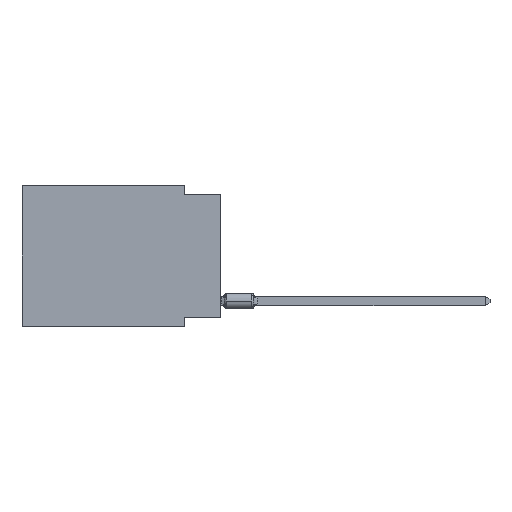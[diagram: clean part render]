
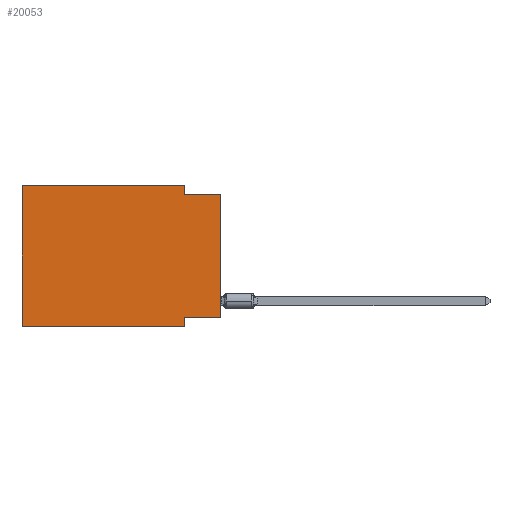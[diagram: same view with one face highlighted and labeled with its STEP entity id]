
A CAD part, left-side view. The second image highlights one B-rep face of the part: STEP entity #20053.
In plain terms, the highlighted planar face has unit normal (-1, 0, 0).
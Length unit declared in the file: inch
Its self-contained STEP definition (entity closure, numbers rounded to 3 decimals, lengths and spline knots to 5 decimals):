
#41 = EDGE_CURVE ( 'NONE', #33202, #29079, #17426, .T. ) ;
#265 = LINE ( 'NONE', #12727, #940 ) ;
#940 = VECTOR ( 'NONE', #28941, 39.37008 ) ;
#988 = CARTESIAN_POINT ( 'NONE',  ( 0., 0., -0.025 ) ) ;
#1193 = VECTOR ( 'NONE', #3491, 39.37008 ) ;
#2106 = AXIS2_PLACEMENT_3D ( 'NONE', #7071, #19017, #40010 ) ;
#3491 = DIRECTION ( 'NONE',  ( 0., 1., 0. ) ) ;
#4586 = VERTEX_POINT ( 'NONE', #39577 ) ;
#5908 = CARTESIAN_POINT ( 'NONE',  ( 0., 0., 0. ) ) ;
#7071 = CARTESIAN_POINT ( 'NONE',  ( 0., 0.55, 0. ) ) ;
#7838 = ORIENTED_EDGE ( 'NONE', *, *, #26029, .F. ) ;
#7906 = ORIENTED_EDGE ( 'NONE', *, *, #47358, .T. ) ;
#8209 = VERTEX_POINT ( 'NONE', #19901 ) ;
#10557 = DIRECTION ( 'NONE',  ( 0., -1., 0. ) ) ;
#10739 = CARTESIAN_POINT ( 'NONE',  ( 0., 0.1, -0.025 ) ) ;
#11230 = EDGE_CURVE ( 'NONE', #8209, #22387, #38913, .T. ) ;
#11458 = VECTOR ( 'NONE', #20767, 39.37008 ) ;
#12727 = CARTESIAN_POINT ( 'NONE',  ( 0., 0.1, 0. ) ) ;
#13503 = VECTOR ( 'NONE', #10557, 39.37008 ) ;
#15391 = EDGE_CURVE ( 'NONE', #31504, #23807, #30764, .T. ) ;
#16105 = VECTOR ( 'NONE', #34143, 39.37008 ) ;
#16266 = CARTESIAN_POINT ( 'NONE',  ( 0., 0.55, -0.39 ) ) ;
#17426 = LINE ( 'NONE', #988, #40096 ) ;
#17578 = DIRECTION ( 'NONE',  ( 0., 0., 1. ) ) ;
#19017 = DIRECTION ( 'NONE',  ( 1., 0., 0. ) ) ;
#19901 = CARTESIAN_POINT ( 'NONE',  ( 0., 0.55, 0. ) ) ;
#19942 = LINE ( 'NONE', #40395, #1193 ) ;
#20053 = ADVANCED_FACE ( 'NONE', ( #27281 ), #23029, .F. ) ;
#20767 = DIRECTION ( 'NONE',  ( 0., 0., 1. ) ) ;
#22218 = CARTESIAN_POINT ( 'NONE',  ( 0., 0.1, -0.39 ) ) ;
#22387 = VERTEX_POINT ( 'NONE', #44448 ) ;
#23029 = PLANE ( 'NONE',  #2106 ) ;
#23807 = VERTEX_POINT ( 'NONE', #52508 ) ;
#24444 = ORIENTED_EDGE ( 'NONE', *, *, #41, .F. ) ;
#25824 = LINE ( 'NONE', #5908, #42724 ) ;
#26029 = EDGE_CURVE ( 'NONE', #4586, #26253, #19942, .T. ) ;
#26253 = VERTEX_POINT ( 'NONE', #43676 ) ;
#27281 = FACE_OUTER_BOUND ( 'NONE', #33804, .T. ) ;
#28511 = CARTESIAN_POINT ( 'NONE',  ( 0., 0., -0.025 ) ) ;
#28941 = DIRECTION ( 'NONE',  ( 0., 0., -1. ) ) ;
#29079 = VERTEX_POINT ( 'NONE', #28511 ) ;
#30367 = EDGE_CURVE ( 'NONE', #31504, #8209, #37250, .T. ) ;
#30508 = CARTESIAN_POINT ( 'NONE',  ( 0., 0.55, -0.39 ) ) ;
#30764 = LINE ( 'NONE', #30508, #13503 ) ;
#31504 = VERTEX_POINT ( 'NONE', #16266 ) ;
#33202 = VERTEX_POINT ( 'NONE', #10739 ) ;
#33263 = ORIENTED_EDGE ( 'NONE', *, *, #15391, .T. ) ;
#33804 = EDGE_LOOP ( 'NONE', ( #7906, #24444, #36402, #45038, #39107, #33263, #42255, #7838 ) ) ;
#34143 = DIRECTION ( 'NONE',  ( 0., -1., 0. ) ) ;
#35199 = VECTOR ( 'NONE', #38928, 39.37008 ) ;
#36402 = ORIENTED_EDGE ( 'NONE', *, *, #41595, .F. ) ;
#37113 = DIRECTION ( 'NONE',  ( 0., -1., 0. ) ) ;
#37250 = LINE ( 'NONE', #44949, #11458 ) ;
#38647 = CARTESIAN_POINT ( 'NONE',  ( 0., 0.55, 0. ) ) ;
#38913 = LINE ( 'NONE', #38647, #16105 ) ;
#38928 = DIRECTION ( 'NONE',  ( 0., 0., -1. ) ) ;
#39107 = ORIENTED_EDGE ( 'NONE', *, *, #30367, .F. ) ;
#39190 = LINE ( 'NONE', #22218, #35199 ) ;
#39577 = CARTESIAN_POINT ( 'NONE',  ( 0., 0., -0.365 ) ) ;
#40010 = DIRECTION ( 'NONE',  ( 0., 0., -1. ) ) ;
#40096 = VECTOR ( 'NONE', #37113, 39.37008 ) ;
#40395 = CARTESIAN_POINT ( 'NONE',  ( 0., 0., -0.365 ) ) ;
#41595 = EDGE_CURVE ( 'NONE', #22387, #33202, #265, .T. ) ;
#42255 = ORIENTED_EDGE ( 'NONE', *, *, #49797, .F. ) ;
#42724 = VECTOR ( 'NONE', #17578, 39.37008 ) ;
#43676 = CARTESIAN_POINT ( 'NONE',  ( 0., 0.1, -0.365 ) ) ;
#44448 = CARTESIAN_POINT ( 'NONE',  ( 0., 0.1, 0. ) ) ;
#44949 = CARTESIAN_POINT ( 'NONE',  ( 0., 0.55, 0. ) ) ;
#45038 = ORIENTED_EDGE ( 'NONE', *, *, #11230, .F. ) ;
#47358 = EDGE_CURVE ( 'NONE', #4586, #29079, #25824, .T. ) ;
#49797 = EDGE_CURVE ( 'NONE', #26253, #23807, #39190, .T. ) ;
#52508 = CARTESIAN_POINT ( 'NONE',  ( 0., 0.1, -0.39 ) ) ;
